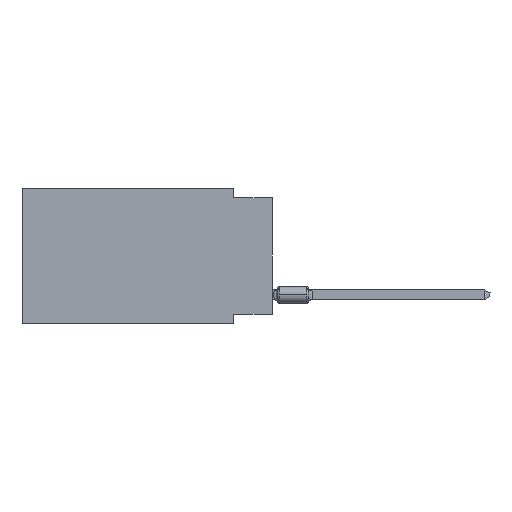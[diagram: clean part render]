
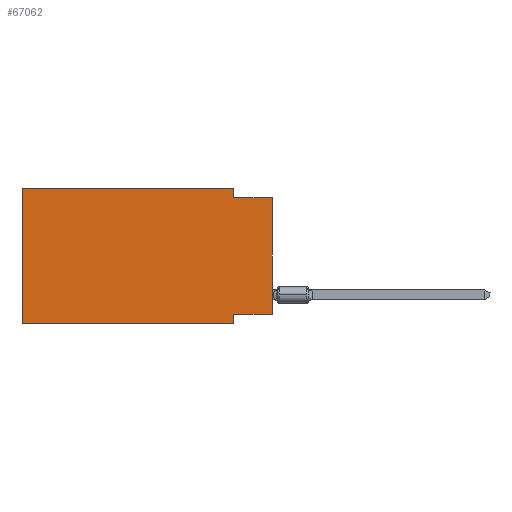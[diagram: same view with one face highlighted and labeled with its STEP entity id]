
A CAD part, left-side view. The second image highlights one B-rep face of the part: STEP entity #67062.
In plain terms, the highlighted planar face has unit normal (-1, 0, 0).
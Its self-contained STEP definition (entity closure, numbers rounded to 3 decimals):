
#647 = CARTESIAN_POINT ( 'NONE',  ( 0., 0., 0. ) ) ;
#2309 = CARTESIAN_POINT ( 'NONE',  ( 0., 16.383, 0. ) ) ;
#3700 = EDGE_CURVE ( 'NONE', #59102, #109866, #42069, .T. ) ;
#4015 = PLANE ( 'NONE',  #96655 ) ;
#7638 = CARTESIAN_POINT ( 'NONE',  ( 0., 0., -8.255 ) ) ;
#9212 = CARTESIAN_POINT ( 'NONE',  ( 0., 16.383, 0. ) ) ;
#9480 = VECTOR ( 'NONE', #40651, 1000. ) ;
#10582 = EDGE_CURVE ( 'NONE', #90490, #93912, #103890, .T. ) ;
#11497 = CARTESIAN_POINT ( 'NONE',  ( 0., 16.383, -8.89 ) ) ;
#12232 = VERTEX_POINT ( 'NONE', #80156 ) ;
#13483 = EDGE_CURVE ( 'NONE', #47703, #12232, #80174, .T. ) ;
#13891 = EDGE_CURVE ( 'NONE', #70563, #53982, #62605, .T. ) ;
#19342 = EDGE_CURVE ( 'NONE', #47703, #90490, #67020, .T. ) ;
#23275 = ORIENTED_EDGE ( 'NONE', *, *, #10582, .F. ) ;
#24051 = EDGE_CURVE ( 'NONE', #70563, #93912, #37639, .T. ) ;
#26757 = CARTESIAN_POINT ( 'NONE',  ( 0., 16.383, 0. ) ) ;
#28271 = EDGE_CURVE ( 'NONE', #53982, #59102, #104553, .T. ) ;
#31318 = EDGE_CURVE ( 'NONE', #109866, #12232, #76978, .T. ) ;
#35472 = DIRECTION ( 'NONE',  ( 0., -1., 0. ) ) ;
#37105 = ORIENTED_EDGE ( 'NONE', *, *, #3700, .F. ) ;
#37639 = LINE ( 'NONE', #11497, #67575 ) ;
#39443 = CARTESIAN_POINT ( 'NONE',  ( 0., 16.383, 0. ) ) ;
#40651 = DIRECTION ( 'NONE',  ( 0., 0., -1. ) ) ;
#41909 = ORIENTED_EDGE ( 'NONE', *, *, #24051, .T. ) ;
#42069 = LINE ( 'NONE', #113449, #108468 ) ;
#44194 = DIRECTION ( 'NONE',  ( 0., 0., 1. ) ) ;
#47561 = DIRECTION ( 'NONE',  ( 1., 0., 0. ) ) ;
#47703 = VERTEX_POINT ( 'NONE', #73010 ) ;
#49700 = DIRECTION ( 'NONE',  ( 0., -1., 0. ) ) ;
#51611 = CARTESIAN_POINT ( 'NONE',  ( 0., 2.54, 0. ) ) ;
#53982 = VERTEX_POINT ( 'NONE', #2309 ) ;
#54482 = DIRECTION ( 'NONE',  ( 0., -1., 0. ) ) ;
#55060 = VECTOR ( 'NONE', #88170, 1000. ) ;
#57595 = VECTOR ( 'NONE', #67597, 1000. ) ;
#59102 = VERTEX_POINT ( 'NONE', #51611 ) ;
#60104 = CARTESIAN_POINT ( 'NONE',  ( 0., 16.383, -8.89 ) ) ;
#60577 = CARTESIAN_POINT ( 'NONE',  ( 0., 2.54, -8.89 ) ) ;
#62023 = ORIENTED_EDGE ( 'NONE', *, *, #19342, .F. ) ;
#62605 = LINE ( 'NONE', #9212, #55060 ) ;
#67020 = LINE ( 'NONE', #7638, #57595 ) ;
#67062 = ADVANCED_FACE ( 'NONE', ( #90549 ), #4015, .F. ) ;
#67232 = ORIENTED_EDGE ( 'NONE', *, *, #13483, .T. ) ;
#67575 = VECTOR ( 'NONE', #54482, 1000. ) ;
#67597 = DIRECTION ( 'NONE',  ( 0., 1., 0. ) ) ;
#70563 = VERTEX_POINT ( 'NONE', #60104 ) ;
#72493 = VECTOR ( 'NONE', #49700, 1000. ) ;
#73010 = CARTESIAN_POINT ( 'NONE',  ( 0., 0., -8.255 ) ) ;
#75721 = VECTOR ( 'NONE', #35472, 1000. ) ;
#76978 = LINE ( 'NONE', #112383, #72493 ) ;
#77772 = ORIENTED_EDGE ( 'NONE', *, *, #13891, .F. ) ;
#80156 = CARTESIAN_POINT ( 'NONE',  ( 0., 0., -0.635 ) ) ;
#80174 = LINE ( 'NONE', #647, #82812 ) ;
#80798 = EDGE_LOOP ( 'NONE', ( #67232, #98688, #37105, #90623, #77772, #41909, #23275, #62023 ) ) ;
#82812 = VECTOR ( 'NONE', #44194, 1000. ) ;
#88170 = DIRECTION ( 'NONE',  ( 0., 0., 1. ) ) ;
#89981 = DIRECTION ( 'NONE',  ( 0., 0., -1. ) ) ;
#90490 = VERTEX_POINT ( 'NONE', #101080 ) ;
#90549 = FACE_OUTER_BOUND ( 'NONE', #80798, .T. ) ;
#90623 = ORIENTED_EDGE ( 'NONE', *, *, #28271, .F. ) ;
#93454 = CARTESIAN_POINT ( 'NONE',  ( 0., 2.54, -8.89 ) ) ;
#93912 = VERTEX_POINT ( 'NONE', #60577 ) ;
#96655 = AXIS2_PLACEMENT_3D ( 'NONE', #39443, #47561, #89981 ) ;
#98688 = ORIENTED_EDGE ( 'NONE', *, *, #31318, .F. ) ;
#101080 = CARTESIAN_POINT ( 'NONE',  ( 0., 2.54, -8.255 ) ) ;
#103890 = LINE ( 'NONE', #93454, #9480 ) ;
#104553 = LINE ( 'NONE', #26757, #75721 ) ;
#104560 = CARTESIAN_POINT ( 'NONE',  ( 0., 2.54, -0.635 ) ) ;
#105884 = DIRECTION ( 'NONE',  ( 0., 0., -1. ) ) ;
#108468 = VECTOR ( 'NONE', #105884, 1000. ) ;
#109866 = VERTEX_POINT ( 'NONE', #104560 ) ;
#112383 = CARTESIAN_POINT ( 'NONE',  ( 0., 0., -0.635 ) ) ;
#113449 = CARTESIAN_POINT ( 'NONE',  ( 0., 2.54, 0. ) ) ;
